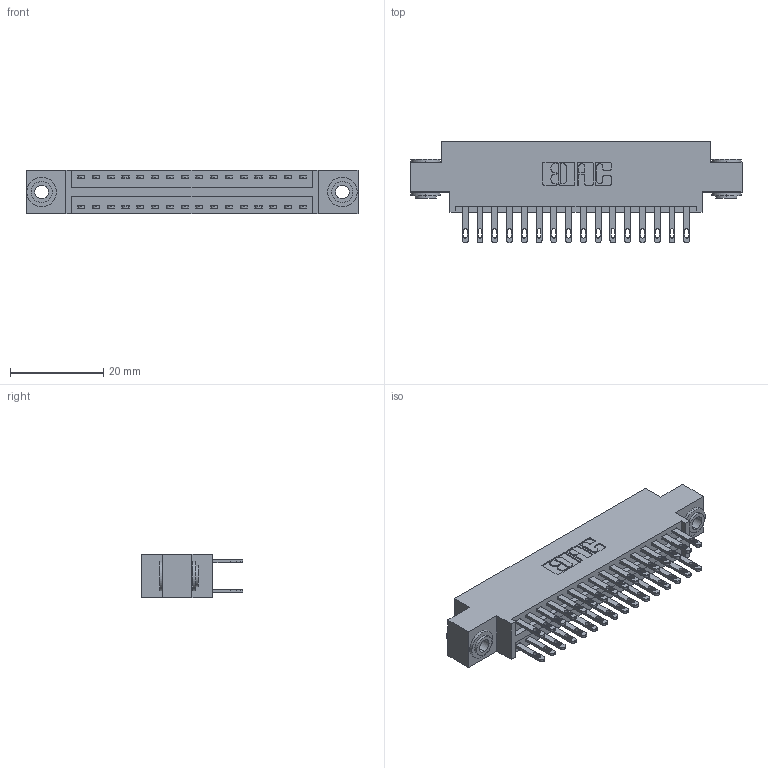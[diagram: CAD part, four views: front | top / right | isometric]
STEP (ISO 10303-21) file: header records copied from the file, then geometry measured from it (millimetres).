
FILE_DESCRIPTION (( 'STEP AP203' ), '1' );
FILE_NAME ('896-032-500-803.STEP', '2021-07-27T19:23:07', ( '' ), ( '' ), 'SwSTEP 2.0', 'SolidWorks 2020', '' );
FILE_SCHEMA (( 'CONFIG_CONTROL_DESIGN' ));
Length unit declared in the file: inch
Products named in the file (4): 345-292-001_345-293-100; 345-250-002_345-250-002-102; 896-032-500-803; 846 Part_0.170 Offset - 0.156 Dia-TH
Assembly tree (35 placements, depth 2):
  896-032-500-803
    846 Part_0.170 Offset - 0.156 Dia-TH
    345-292-001_345-293-100  x32
    345-250-002_345-250-002-102  x2
Bounding box: 71.37 x 21.84 x 9.4 mm (x, y, z)
Volume: 6720.5 mm3; surface area: 9557.8 mm2
Topology: 35 solids, 35 shells, 1700 faces, 5121 edges, 3410 vertices
Faces by surface type: plane 1018, cylinder 674, cone 8
Entity records: 14654 total; most frequent: CARTESIAN_POINT 2427, ORIENTED_EDGE 2354, DIRECTION 2223, EDGE_CURVE 1177, LINE 953, VECTOR 953, VERTEX_POINT 782, AXIS2_PLACEMENT_3D 635
